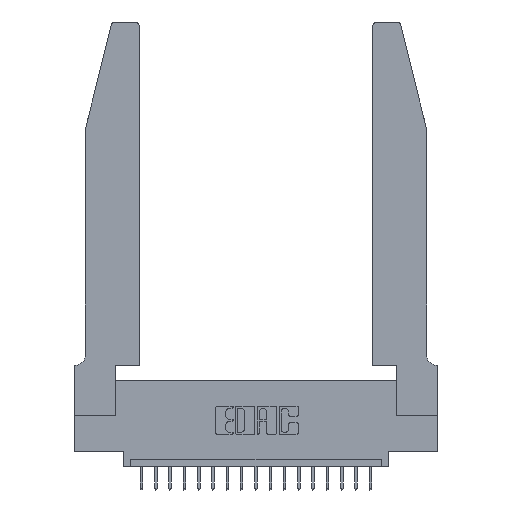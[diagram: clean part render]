
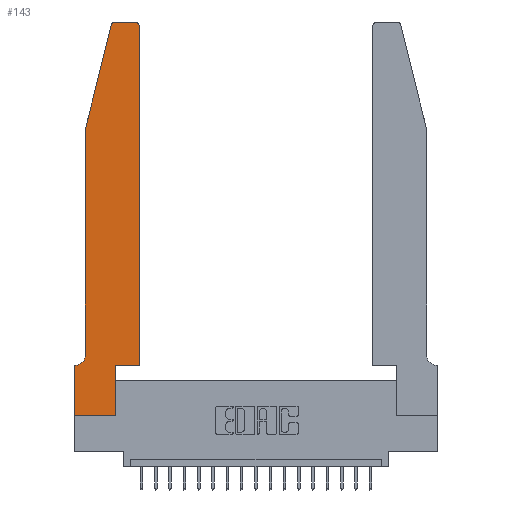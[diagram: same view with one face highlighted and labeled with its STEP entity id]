
A CAD part, top view. The second image highlights one B-rep face of the part: STEP entity #143.
In plain terms, the highlighted planar face has unit normal (0, 0, 1).
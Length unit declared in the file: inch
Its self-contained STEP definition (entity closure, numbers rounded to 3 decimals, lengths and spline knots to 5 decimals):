
#124 = LINE ( 'NONE', #10340, #11836 ) ;
#143 = ADVANCED_FACE ( 'NONE', ( #16166 ), #377, .T. ) ;
#153 = DIRECTION ( 'NONE',  ( 0., 0., 1. ) ) ;
#203 = CARTESIAN_POINT ( 'NONE',  ( 0.2865, 0.35, 0.37 ) ) ;
#218 = VECTOR ( 'NONE', #1943, 39.37008 ) ;
#229 = VERTEX_POINT ( 'NONE', #6710 ) ;
#296 = VERTEX_POINT ( 'NONE', #13391 ) ;
#337 = VECTOR ( 'NONE', #2061, 39.37008 ) ;
#359 = CARTESIAN_POINT ( 'NONE',  ( 0.0055, 0.35, 0.37 ) ) ;
#377 = PLANE ( 'NONE',  #15929 ) ;
#457 = DIRECTION ( 'NONE',  ( 1., 0., 0. ) ) ;
#717 = EDGE_CURVE ( 'NONE', #8973, #14263, #16895, .T. ) ;
#1145 = AXIS2_PLACEMENT_3D ( 'NONE', #13215, #5233, #3455 ) ;
#1943 = DIRECTION ( 'NONE',  ( 0., -1., 0. ) ) ;
#2061 = DIRECTION ( 'NONE',  ( 0., 1., 0. ) ) ;
#2094 = DIRECTION ( 'NONE',  ( 0., 0., 1. ) ) ;
#2670 = EDGE_CURVE ( 'NONE', #20383, #4887, #20153, .T. ) ;
#2861 = LINE ( 'NONE', #19398, #8722 ) ;
#2983 = CARTESIAN_POINT ( 'NONE',  ( 0., 0.35, 0.37 ) ) ;
#3359 = VERTEX_POINT ( 'NONE', #359 ) ;
#3455 = DIRECTION ( 'NONE',  ( -1., 0., 0. ) ) ;
#3516 = AXIS2_PLACEMENT_3D ( 'NONE', #15013, #153, #9963 ) ;
#3641 = EDGE_CURVE ( 'NONE', #3359, #9014, #11091, .T. ) ;
#3810 = VECTOR ( 'NONE', #16663, 39.37008 ) ;
#4459 = CARTESIAN_POINT ( 'NONE',  ( 0.4505, 2.72, 0.37 ) ) ;
#4702 = ORIENTED_EDGE ( 'NONE', *, *, #17811, .T. ) ;
#4887 = VERTEX_POINT ( 'NONE', #11523 ) ;
#5011 = CARTESIAN_POINT ( 'NONE',  ( 0., 0., 0.37 ) ) ;
#5104 = ORIENTED_EDGE ( 'NONE', *, *, #14308, .T. ) ;
#5233 = DIRECTION ( 'NONE',  ( 0., 0., -1. ) ) ;
#5426 = ORIENTED_EDGE ( 'NONE', *, *, #3641, .T. ) ;
#5792 = ORIENTED_EDGE ( 'NONE', *, *, #717, .T. ) ;
#5818 = VECTOR ( 'NONE', #20654, 39.37008 ) ;
#5829 = ORIENTED_EDGE ( 'NONE', *, *, #2670, .T. ) ;
#6341 = CARTESIAN_POINT ( 'NONE',  ( 0., 0., 0.37 ) ) ;
#6710 = CARTESIAN_POINT ( 'NONE',  ( 0.4505, 0.35, 0.37 ) ) ;
#7576 = EDGE_CURVE ( 'NONE', #10486, #3359, #18353, .T. ) ;
#8146 = EDGE_CURVE ( 'NONE', #9014, #20383, #17546, .T. ) ;
#8217 = DIRECTION ( 'NONE',  ( 0., 0., 1. ) ) ;
#8721 = ORIENTED_EDGE ( 'NONE', *, *, #19051, .T. ) ;
#8722 = VECTOR ( 'NONE', #20819, 39.37008 ) ;
#8973 = VERTEX_POINT ( 'NONE', #20969 ) ;
#9014 = VERTEX_POINT ( 'NONE', #2983 ) ;
#9128 = ORIENTED_EDGE ( 'NONE', *, *, #9598, .T. ) ;
#9220 = DIRECTION ( 'NONE',  ( -0.239, -0.971, 0. ) ) ;
#9598 = EDGE_CURVE ( 'NONE', #14263, #296, #13031, .T. ) ;
#9717 = VERTEX_POINT ( 'NONE', #4459 ) ;
#9963 = DIRECTION ( 'NONE',  ( 1., 0., 0. ) ) ;
#10099 = CIRCLE ( 'NONE', #10971, 0.03 ) ;
#10340 = CARTESIAN_POINT ( 'NONE',  ( 0.4505, 0.35, 0.37 ) ) ;
#10343 = CARTESIAN_POINT ( 'NONE',  ( 0.4205, 2.72, 0.37 ) ) ;
#10456 = VECTOR ( 'NONE', #9220, 39.37008 ) ;
#10486 = VERTEX_POINT ( 'NONE', #17924 ) ;
#10573 = CARTESIAN_POINT ( 'NONE',  ( 0.0755, 2., 0.37 ) ) ;
#10815 = ORIENTED_EDGE ( 'NONE', *, *, #14919, .T. ) ;
#10829 = VECTOR ( 'NONE', #19284, 39.37008 ) ;
#10971 = AXIS2_PLACEMENT_3D ( 'NONE', #10343, #2094, #457 ) ;
#11091 = LINE ( 'NONE', #11409, #10829 ) ;
#11409 = CARTESIAN_POINT ( 'NONE',  ( 0.0755, 0.35, 0.37 ) ) ;
#11523 = CARTESIAN_POINT ( 'NONE',  ( 0.2865, 0., 0.37 ) ) ;
#11574 = VERTEX_POINT ( 'NONE', #13343 ) ;
#11836 = VECTOR ( 'NONE', #18575, 39.37008 ) ;
#13031 = LINE ( 'NONE', #10573, #10456 ) ;
#13034 = EDGE_LOOP ( 'NONE', ( #20624, #5792, #9128, #19879, #17937, #5426, #18197, #5829, #4702, #5104, #10815, #8721 ) ) ;
#13215 = CARTESIAN_POINT ( 'NONE',  ( 0.0055, 0.42, 0.37 ) ) ;
#13320 = LINE ( 'NONE', #19837, #337 ) ;
#13343 = CARTESIAN_POINT ( 'NONE',  ( 0.4205, 2.75, 0.37 ) ) ;
#13391 = CARTESIAN_POINT ( 'NONE',  ( 0.0755, 2., 0.37 ) ) ;
#13583 = CARTESIAN_POINT ( 'NONE',  ( 0., 0., 0.37 ) ) ;
#13701 = VECTOR ( 'NONE', #16501, 39.37008 ) ;
#14229 = LINE ( 'NONE', #18536, #5818 ) ;
#14263 = VERTEX_POINT ( 'NONE', #16058 ) ;
#14308 = EDGE_CURVE ( 'NONE', #18888, #229, #124, .T. ) ;
#14919 = EDGE_CURVE ( 'NONE', #229, #9717, #13320, .T. ) ;
#15013 = CARTESIAN_POINT ( 'NONE',  ( 0.284, 2.72, 0.37 ) ) ;
#15290 = EDGE_CURVE ( 'NONE', #296, #10486, #2861, .T. ) ;
#15929 = AXIS2_PLACEMENT_3D ( 'NONE', #18004, #8217, #16474 ) ;
#16058 = CARTESIAN_POINT ( 'NONE',  ( 0.25487, 2.72718, 0.37 ) ) ;
#16166 = FACE_OUTER_BOUND ( 'NONE', #13034, .T. ) ;
#16474 = DIRECTION ( 'NONE',  ( 1., 0., 0. ) ) ;
#16501 = DIRECTION ( 'NONE',  ( 0., 1., 0. ) ) ;
#16663 = DIRECTION ( 'NONE',  ( 1., 0., 0. ) ) ;
#16895 = CIRCLE ( 'NONE', #3516, 0.03 ) ;
#17534 = EDGE_CURVE ( 'NONE', #11574, #8973, #14229, .T. ) ;
#17535 = CARTESIAN_POINT ( 'NONE',  ( 0.2865, 0.35, 0.37 ) ) ;
#17546 = LINE ( 'NONE', #5011, #218 ) ;
#17811 = EDGE_CURVE ( 'NONE', #4887, #18888, #18835, .T. ) ;
#17924 = CARTESIAN_POINT ( 'NONE',  ( 0.0755, 0.42, 0.37 ) ) ;
#17937 = ORIENTED_EDGE ( 'NONE', *, *, #7576, .T. ) ;
#18004 = CARTESIAN_POINT ( 'NONE',  ( 0., 0.35, 0.37 ) ) ;
#18197 = ORIENTED_EDGE ( 'NONE', *, *, #8146, .T. ) ;
#18353 = CIRCLE ( 'NONE', #1145, 0.07 ) ;
#18536 = CARTESIAN_POINT ( 'NONE',  ( 0.2605, 2.75, 0.37 ) ) ;
#18575 = DIRECTION ( 'NONE',  ( 1., 0., 0. ) ) ;
#18835 = LINE ( 'NONE', #203, #13701 ) ;
#18888 = VERTEX_POINT ( 'NONE', #17535 ) ;
#19051 = EDGE_CURVE ( 'NONE', #9717, #11574, #10099, .T. ) ;
#19284 = DIRECTION ( 'NONE',  ( -1., 0., 0. ) ) ;
#19398 = CARTESIAN_POINT ( 'NONE',  ( 0.0755, 2., 0.37 ) ) ;
#19837 = CARTESIAN_POINT ( 'NONE',  ( 0.4505, 0.35, 0.37 ) ) ;
#19879 = ORIENTED_EDGE ( 'NONE', *, *, #15290, .T. ) ;
#20153 = LINE ( 'NONE', #13583, #3810 ) ;
#20383 = VERTEX_POINT ( 'NONE', #6341 ) ;
#20624 = ORIENTED_EDGE ( 'NONE', *, *, #17534, .T. ) ;
#20654 = DIRECTION ( 'NONE',  ( -1., 0., 0. ) ) ;
#20819 = DIRECTION ( 'NONE',  ( 0., -1., 0. ) ) ;
#20969 = CARTESIAN_POINT ( 'NONE',  ( 0.284, 2.75, 0.37 ) ) ;
